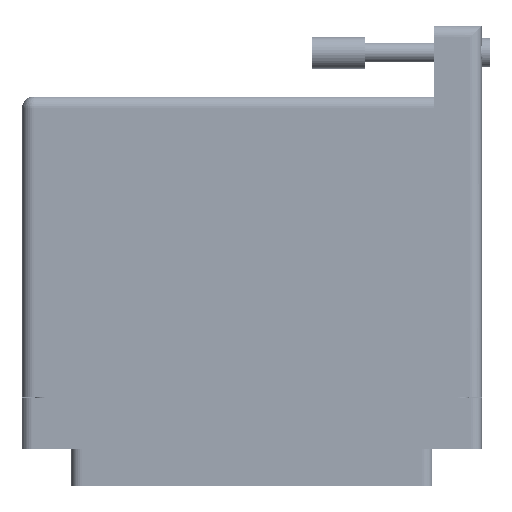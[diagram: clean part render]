
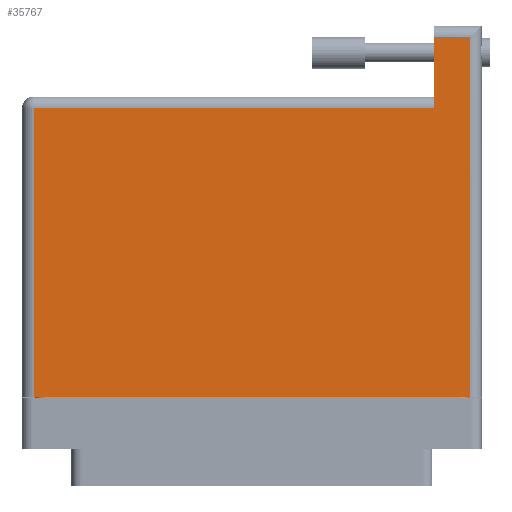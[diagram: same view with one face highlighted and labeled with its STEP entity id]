
A CAD part, front view. The second image highlights one B-rep face of the part: STEP entity #35767.
In plain terms, the highlighted face is planar.
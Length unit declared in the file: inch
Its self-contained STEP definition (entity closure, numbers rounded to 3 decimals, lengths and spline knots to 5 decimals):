
#921 = EDGE_CURVE ( 'NONE', #20011, #30191, #46667, .T. ) ;
#2119 = EDGE_CURVE ( 'NONE', #28702, #64523, #26987, .T. ) ;
#2383 = ORIENTED_EDGE ( 'NONE', *, *, #2119, .T. ) ;
#2925 = DIRECTION ( 'NONE',  ( -1., 0., 0. ) ) ;
#4982 = DIRECTION ( 'NONE',  ( -1., 0., 0. ) ) ;
#4998 = CARTESIAN_POINT ( 'NONE',  ( -1.289, 1.605, 0.617 ) ) ;
#6210 = CARTESIAN_POINT ( 'NONE',  ( 1.079, 2.095, 0.617 ) ) ;
#11582 = EDGE_CURVE ( 'NONE', #64523, #38625, #57267, .T. ) ;
#12385 = EDGE_CURVE ( 'NONE', #30191, #32353, #33996, .T. ) ;
#14510 = CARTESIAN_POINT ( 'NONE',  ( 1.289, 2.025, 0.617 ) ) ;
#15702 = FACE_OUTER_BOUND ( 'NONE', #61805, .T. ) ;
#16986 = AXIS2_PLACEMENT_3D ( 'NONE', #73089, #51435, #39883 ) ;
#18688 = DIRECTION ( 'NONE',  ( 0., -1., 0. ) ) ;
#20011 = VERTEX_POINT ( 'NONE', #4998 ) ;
#23541 = DIRECTION ( 'NONE',  ( 1., 0., 0. ) ) ;
#25098 = CARTESIAN_POINT ( 'NONE',  ( 1.289, 2.095, 0.617 ) ) ;
#26987 = LINE ( 'NONE', #56747, #55987 ) ;
#28702 = VERTEX_POINT ( 'NONE', #14510 ) ;
#29135 = ORIENTED_EDGE ( 'NONE', *, *, #12385, .T. ) ;
#30191 = VERTEX_POINT ( 'NONE', #64025 ) ;
#30883 = LINE ( 'NONE', #58098, #64210 ) ;
#31047 = ORIENTED_EDGE ( 'NONE', *, *, #11582, .T. ) ;
#32353 = VERTEX_POINT ( 'NONE', #34840 ) ;
#33996 = LINE ( 'NONE', #51494, #34096 ) ;
#34096 = VECTOR ( 'NONE', #23541, 39.37008 ) ;
#34840 = CARTESIAN_POINT ( 'NONE',  ( 1.289, -0.1, 0.617 ) ) ;
#35767 = ADVANCED_FACE ( 'NONE', ( #15702 ), #56296, .F. ) ;
#38625 = VERTEX_POINT ( 'NONE', #72759 ) ;
#38772 = VECTOR ( 'NONE', #51673, 39.37008 ) ;
#39883 = DIRECTION ( 'NONE',  ( -1., 0., 0. ) ) ;
#40974 = VECTOR ( 'NONE', #70918, 39.37008 ) ;
#41130 = ORIENTED_EDGE ( 'NONE', *, *, #52195, .T. ) ;
#45573 = CARTESIAN_POINT ( 'NONE',  ( -1.289, -0.1, 0.617 ) ) ;
#45830 = EDGE_CURVE ( 'NONE', #38625, #20011, #30883, .T. ) ;
#46667 = LINE ( 'NONE', #45573, #52428 ) ;
#51435 = DIRECTION ( 'NONE',  ( 0., 0., -1. ) ) ;
#51494 = CARTESIAN_POINT ( 'NONE',  ( -1.359, -0.1, 0.617 ) ) ;
#51673 = DIRECTION ( 'NONE',  ( 0., -1., 0. ) ) ;
#52195 = EDGE_CURVE ( 'NONE', #32353, #28702, #58617, .T. ) ;
#52428 = VECTOR ( 'NONE', #18688, 39.37008 ) ;
#53297 = CARTESIAN_POINT ( 'NONE',  ( 1.079, 2.025, 0.617 ) ) ;
#55987 = VECTOR ( 'NONE', #4982, 39.37008 ) ;
#56296 = PLANE ( 'NONE',  #16986 ) ;
#56747 = CARTESIAN_POINT ( 'NONE',  ( -1.359, 2.025, 0.617 ) ) ;
#57267 = LINE ( 'NONE', #6210, #38772 ) ;
#58036 = ORIENTED_EDGE ( 'NONE', *, *, #921, .T. ) ;
#58098 = CARTESIAN_POINT ( 'NONE',  ( -1.359, 1.605, 0.617 ) ) ;
#58617 = LINE ( 'NONE', #25098, #40974 ) ;
#61805 = EDGE_LOOP ( 'NONE', ( #65826, #58036, #29135, #41130, #2383, #31047 ) ) ;
#64025 = CARTESIAN_POINT ( 'NONE',  ( -1.289, -0.1, 0.617 ) ) ;
#64210 = VECTOR ( 'NONE', #2925, 39.37008 ) ;
#64523 = VERTEX_POINT ( 'NONE', #53297 ) ;
#65826 = ORIENTED_EDGE ( 'NONE', *, *, #45830, .T. ) ;
#70918 = DIRECTION ( 'NONE',  ( 0., 1., 0. ) ) ;
#72759 = CARTESIAN_POINT ( 'NONE',  ( 1.079, 1.605, 0.617 ) ) ;
#73089 = CARTESIAN_POINT ( 'NONE',  ( -1.359, 1.675, 0.617 ) ) ;
